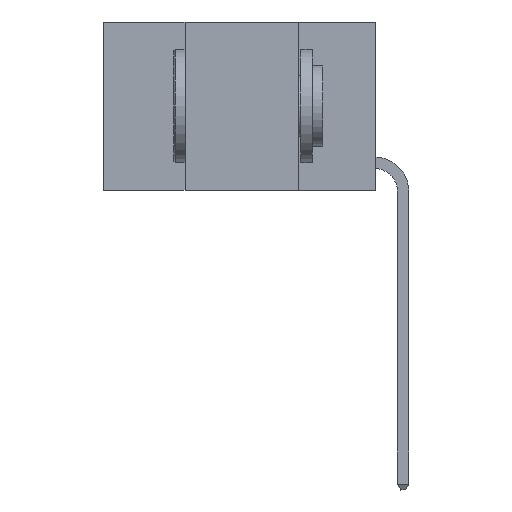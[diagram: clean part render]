
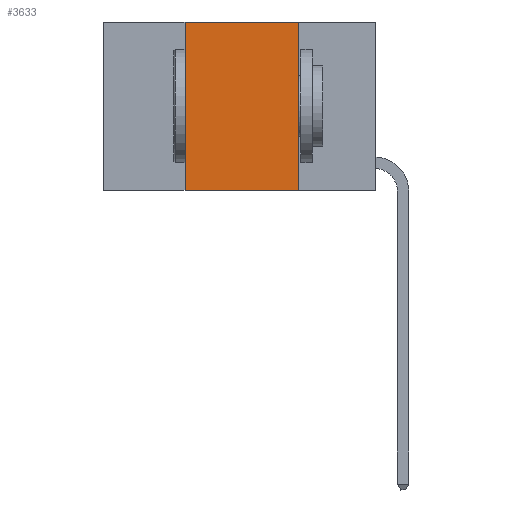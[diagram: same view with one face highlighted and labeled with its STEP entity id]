
A CAD part, left-side view. The second image highlights one B-rep face of the part: STEP entity #3633.
In plain terms, the highlighted planar face has unit normal (-1, 0, 0).
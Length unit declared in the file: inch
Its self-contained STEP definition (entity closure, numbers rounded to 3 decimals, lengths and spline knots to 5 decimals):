
#403 = VECTOR ( 'NONE', #2839, 39.37008 ) ;
#810 = CARTESIAN_POINT ( 'NONE',  ( 0., 0.6, 0. ) ) ;
#1217 = EDGE_LOOP ( 'NONE', ( #20988, #24119, #24481, #16409 ) ) ;
#2839 = DIRECTION ( 'NONE',  ( 0., 0., 1. ) ) ;
#3477 = CARTESIAN_POINT ( 'NONE',  ( 0., 0.6, 0. ) ) ;
#3633 = ADVANCED_FACE ( 'NONE', ( #7394 ), #12389, .F. ) ;
#4526 = AXIS2_PLACEMENT_3D ( 'NONE', #810, #12240, #9536 ) ;
#4650 = VECTOR ( 'NONE', #26410, 39.37008 ) ;
#7394 = FACE_OUTER_BOUND ( 'NONE', #1217, .T. ) ;
#9186 = VERTEX_POINT ( 'NONE', #18519 ) ;
#9536 = DIRECTION ( 'NONE',  ( 0., 0., -1. ) ) ;
#10081 = CARTESIAN_POINT ( 'NONE',  ( 0., 0.17, 0. ) ) ;
#12066 = EDGE_CURVE ( 'NONE', #25836, #23627, #13104, .T. ) ;
#12240 = DIRECTION ( 'NONE',  ( 1., 0., 0. ) ) ;
#12389 = PLANE ( 'NONE',  #4526 ) ;
#12922 = VECTOR ( 'NONE', #21363, 39.37008 ) ;
#13104 = LINE ( 'NONE', #3477, #12922 ) ;
#13970 = LINE ( 'NONE', #22445, #403 ) ;
#16409 = ORIENTED_EDGE ( 'NONE', *, *, #22841, .T. ) ;
#17672 = CARTESIAN_POINT ( 'NONE',  ( 0., 0.6, -0.37 ) ) ;
#18519 = CARTESIAN_POINT ( 'NONE',  ( 0., 0.17, -0.37 ) ) ;
#18812 = LINE ( 'NONE', #10081, #23981 ) ;
#19798 = LINE ( 'NONE', #17672, #4650 ) ;
#20370 = EDGE_CURVE ( 'NONE', #25388, #25836, #13970, .T. ) ;
#20988 = ORIENTED_EDGE ( 'NONE', *, *, #25148, .F. ) ;
#21287 = CARTESIAN_POINT ( 'NONE',  ( 0., 0.17, 0. ) ) ;
#21363 = DIRECTION ( 'NONE',  ( 0., -1., 0. ) ) ;
#22445 = CARTESIAN_POINT ( 'NONE',  ( 0., 0.42, 0. ) ) ;
#22841 = EDGE_CURVE ( 'NONE', #25388, #9186, #19798, .T. ) ;
#23627 = VERTEX_POINT ( 'NONE', #21287 ) ;
#23947 = CARTESIAN_POINT ( 'NONE',  ( 0., 0.42, -0.37 ) ) ;
#23981 = VECTOR ( 'NONE', #27270, 39.37008 ) ;
#24119 = ORIENTED_EDGE ( 'NONE', *, *, #12066, .F. ) ;
#24481 = ORIENTED_EDGE ( 'NONE', *, *, #20370, .F. ) ;
#25148 = EDGE_CURVE ( 'NONE', #23627, #9186, #18812, .T. ) ;
#25388 = VERTEX_POINT ( 'NONE', #23947 ) ;
#25836 = VERTEX_POINT ( 'NONE', #28258 ) ;
#26410 = DIRECTION ( 'NONE',  ( 0., -1., 0. ) ) ;
#27270 = DIRECTION ( 'NONE',  ( 0., 0., -1. ) ) ;
#28258 = CARTESIAN_POINT ( 'NONE',  ( 0., 0.42, 0. ) ) ;
